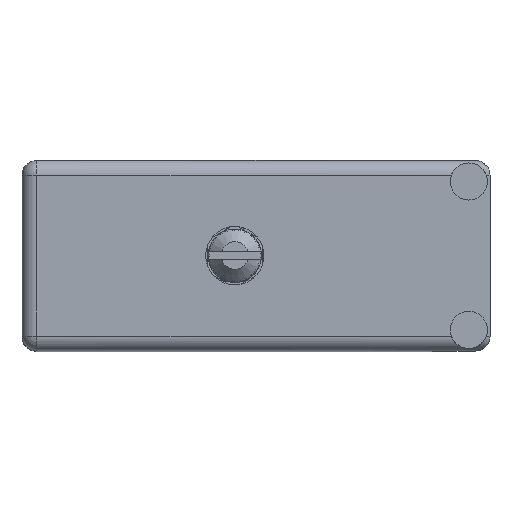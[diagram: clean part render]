
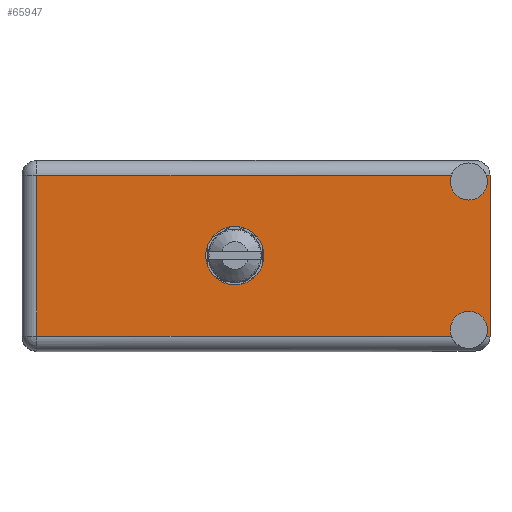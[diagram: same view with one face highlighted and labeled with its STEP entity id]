
A CAD part, top view. The second image highlights one B-rep face of the part: STEP entity #65947.
In plain terms, the highlighted face is planar.
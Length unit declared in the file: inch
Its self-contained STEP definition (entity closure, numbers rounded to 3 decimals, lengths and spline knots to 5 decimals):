
#2835 = VERTEX_POINT ( 'NONE', #80850 ) ;
#3765 = DIRECTION ( 'NONE',  ( 0., 0., 1. ) ) ;
#4517 = VECTOR ( 'NONE', #96221, 39.37008 ) ;
#5075 = DIRECTION ( 'NONE',  ( 0., 0., 1. ) ) ;
#6303 = EDGE_CURVE ( 'NONE', #13247, #69064, #49987, .T. ) ;
#6459 = CARTESIAN_POINT ( 'NONE',  ( -0.934, 1.466, -0.4495 ) ) ;
#7107 = VECTOR ( 'NONE', #102481, 39.37008 ) ;
#7121 = AXIS2_PLACEMENT_3D ( 'NONE', #38745, #63431, #5075 ) ;
#7145 = EDGE_CURVE ( 'NONE', #81085, #11553, #17817, .T. ) ;
#9868 = VERTEX_POINT ( 'NONE', #17690 ) ;
#11553 = VERTEX_POINT ( 'NONE', #22567 ) ;
#13247 = VERTEX_POINT ( 'NONE', #56301 ) ;
#14742 = LINE ( 'NONE', #90362, #94924 ) ;
#14999 = EDGE_CURVE ( 'NONE', #63824, #11553, #14742, .T. ) ;
#16984 = DIRECTION ( 'NONE',  ( 0., 1., 0. ) ) ;
#17025 = CARTESIAN_POINT ( 'NONE',  ( 0., 1.466, -0.1375 ) ) ;
#17690 = CARTESIAN_POINT ( 'NONE',  ( 1.18638, 1.466, -0.3795 ) ) ;
#17729 = EDGE_CURVE ( 'NONE', #67530, #73655, #66555, .T. ) ;
#17817 = LINE ( 'NONE', #66204, #85864 ) ;
#19102 = CARTESIAN_POINT ( 'NONE',  ( 1.18638, 1.466, 0.3795 ) ) ;
#21671 = EDGE_CURVE ( 'NONE', #2835, #41685, #83378, .T. ) ;
#22567 = CARTESIAN_POINT ( 'NONE',  ( 1.204, 1.466, 0.3795 ) ) ;
#23465 = ORIENTED_EDGE ( 'NONE', *, *, #76363, .F. ) ;
#23767 = ORIENTED_EDGE ( 'NONE', *, *, #6303, .F. ) ;
#23971 = CARTESIAN_POINT ( 'NONE',  ( -0.934, 1.466, 0.3795 ) ) ;
#24269 = ORIENTED_EDGE ( 'NONE', *, *, #26880, .F. ) ;
#26880 = EDGE_CURVE ( 'NONE', #73655, #9868, #92244, .T. ) ;
#27390 = CARTESIAN_POINT ( 'NONE',  ( 1.104, 1.466, -0.35 ) ) ;
#32093 = CARTESIAN_POINT ( 'NONE',  ( 1.02162, 1.466, -0.3795 ) ) ;
#32562 = EDGE_LOOP ( 'NONE', ( #23767, #71901 ) ) ;
#32909 = CIRCLE ( 'NONE', #7121, 0.1375 ) ;
#34605 = EDGE_CURVE ( 'NONE', #67139, #41685, #100555, .T. ) ;
#35516 = DIRECTION ( 'NONE',  ( 0., 1., 0. ) ) ;
#36370 = DIRECTION ( 'NONE',  ( 0., 0., 1. ) ) ;
#36420 = CARTESIAN_POINT ( 'NONE',  ( -1.004, 1.466, -0.3795 ) ) ;
#36627 = CARTESIAN_POINT ( 'NONE',  ( -1.004, 1.466, -0.3795 ) ) ;
#37016 = LINE ( 'NONE', #36627, #106511 ) ;
#38203 = CARTESIAN_POINT ( 'NONE',  ( 1.104, 1.466, 0.35 ) ) ;
#38745 = CARTESIAN_POINT ( 'NONE',  ( 0., 1.466, 0. ) ) ;
#41685 = VERTEX_POINT ( 'NONE', #66025 ) ;
#42429 = ORIENTED_EDGE ( 'NONE', *, *, #17729, .F. ) ;
#42466 = AXIS2_PLACEMENT_3D ( 'NONE', #78244, #70487, #61541 ) ;
#43296 = EDGE_CURVE ( 'NONE', #67530, #108935, #91502, .T. ) ;
#43491 = DIRECTION ( 'NONE',  ( -1., 0., 0. ) ) ;
#44596 = DIRECTION ( 'NONE',  ( 0., 1., 0. ) ) ;
#47790 = DIRECTION ( 'NONE',  ( 1., 0., 0. ) ) ;
#48623 = LINE ( 'NONE', #6459, #7107 ) ;
#49293 = CARTESIAN_POINT ( 'NONE',  ( 0., 1.466, 0. ) ) ;
#49987 = CIRCLE ( 'NONE', #53597, 0.1375 ) ;
#52212 = AXIS2_PLACEMENT_3D ( 'NONE', #38203, #98001, #106586 ) ;
#52665 = ORIENTED_EDGE ( 'NONE', *, *, #43296, .T. ) ;
#52796 = AXIS2_PLACEMENT_3D ( 'NONE', #60374, #16984, #43491 ) ;
#53585 = ORIENTED_EDGE ( 'NONE', *, *, #14999, .T. ) ;
#53597 = AXIS2_PLACEMENT_3D ( 'NONE', #49293, #35516, #91812 ) ;
#54605 = CARTESIAN_POINT ( 'NONE',  ( 1.104, 1.466, 0.35 ) ) ;
#55864 = DIRECTION ( 'NONE',  ( 1., 0., 0. ) ) ;
#56141 = DIRECTION ( 'NONE',  ( 0., 0., 1. ) ) ;
#56301 = CARTESIAN_POINT ( 'NONE',  ( 0., 1.466, 0.1375 ) ) ;
#56805 = FACE_OUTER_BOUND ( 'NONE', #94459, .T. ) ;
#56845 = ORIENTED_EDGE ( 'NONE', *, *, #89429, .T. ) ;
#59817 = ORIENTED_EDGE ( 'NONE', *, *, #34605, .T. ) ;
#60204 = CARTESIAN_POINT ( 'NONE',  ( 1.204, 1.466, -0.3795 ) ) ;
#60374 = CARTESIAN_POINT ( 'NONE',  ( -1.004, 1.466, -0.4495 ) ) ;
#60859 = ORIENTED_EDGE ( 'NONE', *, *, #21671, .F. ) ;
#61541 = DIRECTION ( 'NONE',  ( 0., 0., 1. ) ) ;
#63431 = DIRECTION ( 'NONE',  ( 0., 1., 0. ) ) ;
#63824 = VERTEX_POINT ( 'NONE', #19102 ) ;
#65813 = VECTOR ( 'NONE', #55864, 39.37008 ) ;
#65947 = ADVANCED_FACE ( 'NONE', ( #86405, #56805 ), #67827, .T. ) ;
#66025 = CARTESIAN_POINT ( 'NONE',  ( 1.02162, 1.466, 0.3795 ) ) ;
#66204 = CARTESIAN_POINT ( 'NONE',  ( 1.204, 1.466, 0.4495 ) ) ;
#66555 = CIRCLE ( 'NONE', #42466, 0.0875 ) ;
#67139 = VERTEX_POINT ( 'NONE', #23971 ) ;
#67530 = VERTEX_POINT ( 'NONE', #32093 ) ;
#67827 = PLANE ( 'NONE',  #52796 ) ;
#67875 = EDGE_CURVE ( 'NONE', #69064, #13247, #32909, .T. ) ;
#69064 = VERTEX_POINT ( 'NONE', #17025 ) ;
#69774 = ORIENTED_EDGE ( 'NONE', *, *, #77337, .T. ) ;
#70487 = DIRECTION ( 'NONE',  ( 0., 1., 0. ) ) ;
#71901 = ORIENTED_EDGE ( 'NONE', *, *, #67875, .F. ) ;
#73655 = VERTEX_POINT ( 'NONE', #81441 ) ;
#73908 = AXIS2_PLACEMENT_3D ( 'NONE', #54605, #105456, #3765 ) ;
#76363 = EDGE_CURVE ( 'NONE', #63824, #2835, #93414, .T. ) ;
#77337 = EDGE_CURVE ( 'NONE', #108935, #67139, #48623, .T. ) ;
#77888 = AXIS2_PLACEMENT_3D ( 'NONE', #27390, #44596, #36370 ) ;
#78244 = CARTESIAN_POINT ( 'NONE',  ( 1.104, 1.466, -0.35 ) ) ;
#80850 = CARTESIAN_POINT ( 'NONE',  ( 1.104, 1.466, 0.2625 ) ) ;
#81085 = VERTEX_POINT ( 'NONE', #60204 ) ;
#81441 = CARTESIAN_POINT ( 'NONE',  ( 1.104, 1.466, -0.2625 ) ) ;
#83378 = CIRCLE ( 'NONE', #52212, 0.0875 ) ;
#85864 = VECTOR ( 'NONE', #56141, 39.37008 ) ;
#86405 = FACE_BOUND ( 'NONE', #32562, .T. ) ;
#86666 = DIRECTION ( 'NONE',  ( -1., 0., 0. ) ) ;
#89429 = EDGE_CURVE ( 'NONE', #81085, #9868, #37016, .T. ) ;
#90362 = CARTESIAN_POINT ( 'NONE',  ( 1.204, 1.466, 0.3795 ) ) ;
#91502 = LINE ( 'NONE', #36420, #4517 ) ;
#91812 = DIRECTION ( 'NONE',  ( 0., 0., 1. ) ) ;
#92244 = CIRCLE ( 'NONE', #77888, 0.0875 ) ;
#93414 = CIRCLE ( 'NONE', #73908, 0.0875 ) ;
#94459 = EDGE_LOOP ( 'NONE', ( #59817, #60859, #23465, #53585, #109838, #56845, #24269, #42429, #52665, #69774 ) ) ;
#94924 = VECTOR ( 'NONE', #47790, 39.37008 ) ;
#96221 = DIRECTION ( 'NONE',  ( -1., 0., 0. ) ) ;
#98001 = DIRECTION ( 'NONE',  ( 0., 1., 0. ) ) ;
#100555 = LINE ( 'NONE', #107034, #65813 ) ;
#102481 = DIRECTION ( 'NONE',  ( 0., 0., 1. ) ) ;
#105456 = DIRECTION ( 'NONE',  ( 0., 1., 0. ) ) ;
#106511 = VECTOR ( 'NONE', #86666, 39.37008 ) ;
#106586 = DIRECTION ( 'NONE',  ( 0., 0., 1. ) ) ;
#107034 = CARTESIAN_POINT ( 'NONE',  ( 1.204, 1.466, 0.3795 ) ) ;
#108935 = VERTEX_POINT ( 'NONE', #109263 ) ;
#109263 = CARTESIAN_POINT ( 'NONE',  ( -0.934, 1.466, -0.3795 ) ) ;
#109838 = ORIENTED_EDGE ( 'NONE', *, *, #7145, .F. ) ;
